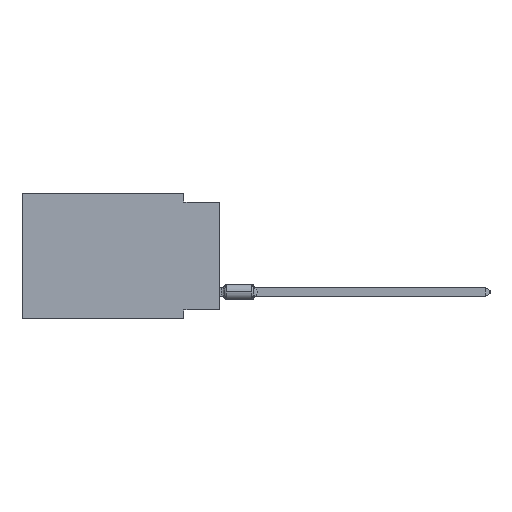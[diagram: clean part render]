
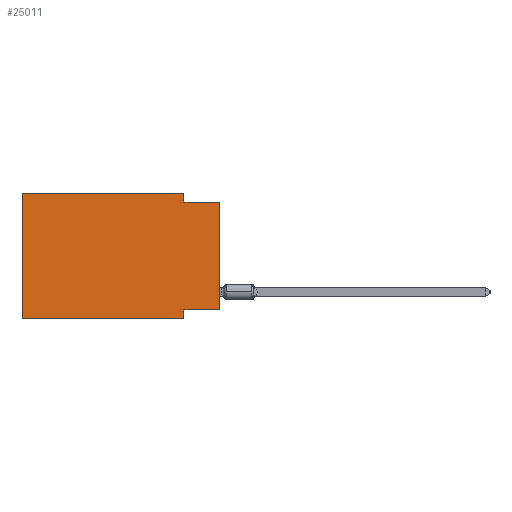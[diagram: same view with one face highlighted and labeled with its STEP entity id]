
A CAD part, left-side view. The second image highlights one B-rep face of the part: STEP entity #25011.
In plain terms, the highlighted planar face has unit normal (-1, 0, 0).
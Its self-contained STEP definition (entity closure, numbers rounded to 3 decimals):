
#621 = DIRECTION ( 'NONE',  ( 0., 1., 0. ) ) ;
#1617 = CARTESIAN_POINT ( 'NONE',  ( 0., 0., -8.255 ) ) ;
#5529 = VERTEX_POINT ( 'NONE', #21699 ) ;
#5943 = CARTESIAN_POINT ( 'NONE',  ( 0., 13.97, -8.89 ) ) ;
#6032 = LINE ( 'NONE', #19432, #22998 ) ;
#6514 = CARTESIAN_POINT ( 'NONE',  ( 0., 13.97, -8.89 ) ) ;
#6937 = EDGE_CURVE ( 'NONE', #32318, #10529, #29762, .T. ) ;
#7608 = ORIENTED_EDGE ( 'NONE', *, *, #36932, .F. ) ;
#8970 = CARTESIAN_POINT ( 'NONE',  ( 0., 13.97, 0. ) ) ;
#9047 = CARTESIAN_POINT ( 'NONE',  ( 0., 2.54, 0. ) ) ;
#9810 = ORIENTED_EDGE ( 'NONE', *, *, #20846, .F. ) ;
#10499 = EDGE_CURVE ( 'NONE', #21550, #5529, #35101, .T. ) ;
#10529 = VERTEX_POINT ( 'NONE', #16782 ) ;
#10726 = VECTOR ( 'NONE', #621, 1000. ) ;
#10798 = DIRECTION ( 'NONE',  ( 0., 0., 1. ) ) ;
#11218 = DIRECTION ( 'NONE',  ( 0., -1., 0. ) ) ;
#12002 = CARTESIAN_POINT ( 'NONE',  ( 0., 2.54, 0. ) ) ;
#13793 = ORIENTED_EDGE ( 'NONE', *, *, #10499, .T. ) ;
#14701 = EDGE_CURVE ( 'NONE', #32318, #36650, #25081, .T. ) ;
#14948 = EDGE_CURVE ( 'NONE', #20436, #36650, #21213, .T. ) ;
#15319 = ORIENTED_EDGE ( 'NONE', *, *, #14948, .F. ) ;
#15775 = DIRECTION ( 'NONE',  ( 0., -1., 0. ) ) ;
#16782 = CARTESIAN_POINT ( 'NONE',  ( 0., 2.54, -8.255 ) ) ;
#18419 = VECTOR ( 'NONE', #18922, 1000. ) ;
#18822 = ORIENTED_EDGE ( 'NONE', *, *, #6937, .F. ) ;
#18892 = VECTOR ( 'NONE', #29225, 1000. ) ;
#18922 = DIRECTION ( 'NONE',  ( 0., -1., 0. ) ) ;
#18941 = EDGE_LOOP ( 'NONE', ( #29464, #15319, #30130, #7608, #9810, #13793, #31572, #18822 ) ) ;
#19096 = VECTOR ( 'NONE', #11218, 1000. ) ;
#19432 = CARTESIAN_POINT ( 'NONE',  ( 0., 13.97, 0. ) ) ;
#20049 = VECTOR ( 'NONE', #10798, 1000. ) ;
#20436 = VERTEX_POINT ( 'NONE', #35859 ) ;
#20719 = LINE ( 'NONE', #23912, #29573 ) ;
#20846 = EDGE_CURVE ( 'NONE', #21550, #27452, #6032, .T. ) ;
#21213 = LINE ( 'NONE', #30984, #19096 ) ;
#21515 = PLANE ( 'NONE',  #37431 ) ;
#21550 = VERTEX_POINT ( 'NONE', #6514 ) ;
#21699 = CARTESIAN_POINT ( 'NONE',  ( 0., 2.54, -8.89 ) ) ;
#22998 = VECTOR ( 'NONE', #35811, 1000. ) ;
#23912 = CARTESIAN_POINT ( 'NONE',  ( 0., 2.54, -8.89 ) ) ;
#25011 = ADVANCED_FACE ( 'NONE', ( #38121 ), #21515, .F. ) ;
#25081 = LINE ( 'NONE', #38062, #20049 ) ;
#27452 = VERTEX_POINT ( 'NONE', #28371 ) ;
#28116 = DIRECTION ( 'NONE',  ( 0., 0., -1. ) ) ;
#28371 = CARTESIAN_POINT ( 'NONE',  ( 0., 13.97, 0. ) ) ;
#28398 = VECTOR ( 'NONE', #15775, 1000. ) ;
#29225 = DIRECTION ( 'NONE',  ( 0., 0., -1. ) ) ;
#29464 = ORIENTED_EDGE ( 'NONE', *, *, #14701, .T. ) ;
#29573 = VECTOR ( 'NONE', #33696, 1000. ) ;
#29762 = LINE ( 'NONE', #39983, #10726 ) ;
#30130 = ORIENTED_EDGE ( 'NONE', *, *, #32390, .F. ) ;
#30984 = CARTESIAN_POINT ( 'NONE',  ( 0., 0., -0.635 ) ) ;
#31572 = ORIENTED_EDGE ( 'NONE', *, *, #33871, .F. ) ;
#32318 = VERTEX_POINT ( 'NONE', #1617 ) ;
#32390 = EDGE_CURVE ( 'NONE', #37598, #20436, #32430, .T. ) ;
#32430 = LINE ( 'NONE', #9047, #18892 ) ;
#33696 = DIRECTION ( 'NONE',  ( 0., 0., -1. ) ) ;
#33871 = EDGE_CURVE ( 'NONE', #10529, #5529, #20719, .T. ) ;
#34725 = CARTESIAN_POINT ( 'NONE',  ( 0., 13.97, 0. ) ) ;
#35101 = LINE ( 'NONE', #5943, #18419 ) ;
#35124 = DIRECTION ( 'NONE',  ( 1., 0., 0. ) ) ;
#35811 = DIRECTION ( 'NONE',  ( 0., 0., 1. ) ) ;
#35859 = CARTESIAN_POINT ( 'NONE',  ( 0., 2.54, -0.635 ) ) ;
#36129 = LINE ( 'NONE', #34725, #28398 ) ;
#36650 = VERTEX_POINT ( 'NONE', #40049 ) ;
#36932 = EDGE_CURVE ( 'NONE', #27452, #37598, #36129, .T. ) ;
#37431 = AXIS2_PLACEMENT_3D ( 'NONE', #8970, #35124, #28116 ) ;
#37598 = VERTEX_POINT ( 'NONE', #12002 ) ;
#38062 = CARTESIAN_POINT ( 'NONE',  ( 0., 0., 0. ) ) ;
#38121 = FACE_OUTER_BOUND ( 'NONE', #18941, .T. ) ;
#39983 = CARTESIAN_POINT ( 'NONE',  ( 0., 0., -8.255 ) ) ;
#40049 = CARTESIAN_POINT ( 'NONE',  ( 0., 0., -0.635 ) ) ;
